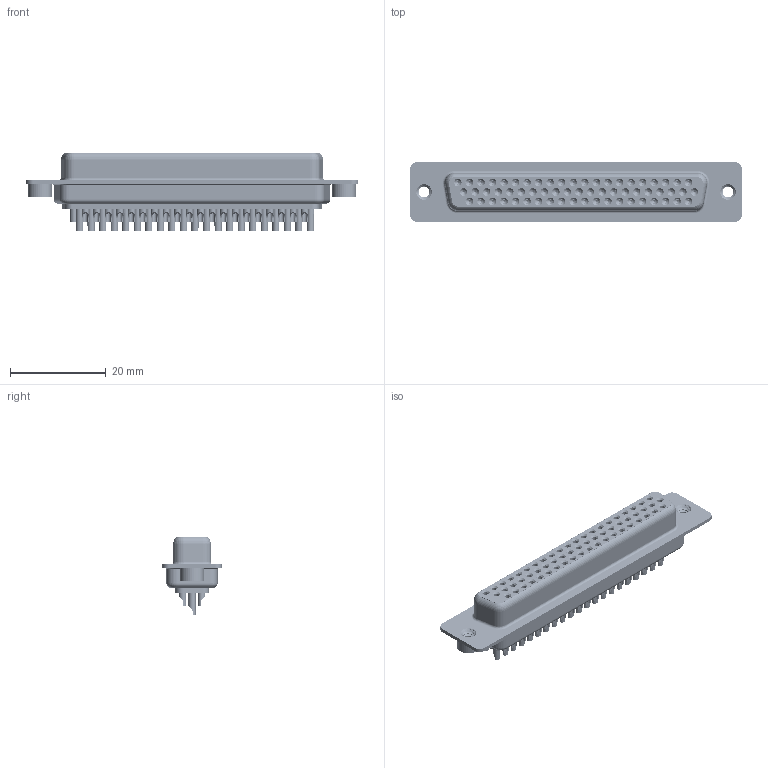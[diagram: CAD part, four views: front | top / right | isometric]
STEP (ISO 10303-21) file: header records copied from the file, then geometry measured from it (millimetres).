
FILE_DESCRIPTION (( 'STEP AP203' ), '1' );
FILE_NAME ('638-M62-232-BT2.STEP', '2022-07-05T21:20:50', ( '' ), ( '' ), 'SwSTEP 2.0', 'SolidWorks 2020', '' );
FILE_SCHEMA (( 'CONFIG_CONTROL_DESIGN' ));
Length unit declared in the file: millimetre
Products named in the file (8): 638M Contact Row 3_32; 638M Housing_62 Contacts; 638-M62-232-BT2; 638M Shell Front_62 Contacts; 638M Shell Rear_62 Contacts; 638M Contact Row 1_32; 638M Contact Row 2_32; 638M 4-40 Threaded Rivet
Assembly tree (67 placements, depth 2):
  638-M62-232-BT2
    638M Housing_62 Contacts
    638M Shell Front_62 Contacts
    638M Shell Rear_62 Contacts
    638M Contact Row 1_32  x21
    638M Contact Row 2_32  x21
    638M Contact Row 3_32  x20
    638M 4-40 Threaded Rivet  x2
Bounding box: 69.4 x 12.5 x 16.45 mm (x, y, z)
Volume: 5073.6 mm3; surface area: 16874.2 mm2
Topology: 67 solids, 67 shells, 3689 faces, 9117 edges, 5635 vertices
Faces by surface type: cylinder 1439, plane 1121, cone 570, torus 553, bspline 6
Entity records: 37914 total; most frequent: CARTESIAN_POINT 7424, DIRECTION 6544, ORIENTED_EDGE 5304, AXIS2_PLACEMENT_3D 2778, EDGE_CURVE 2652, VERTEX_POINT 1689, CIRCLE 1533, EDGE_LOOP 1517
